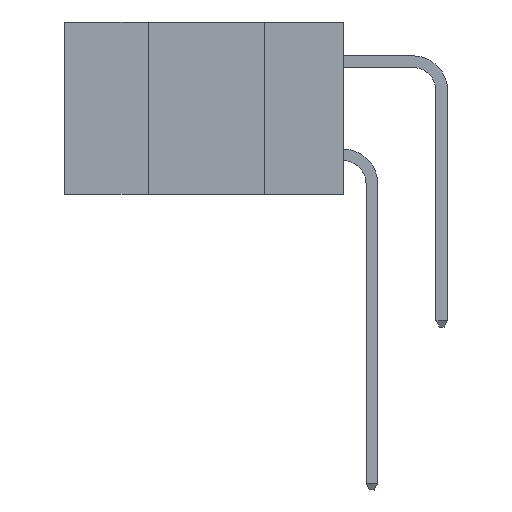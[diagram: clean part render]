
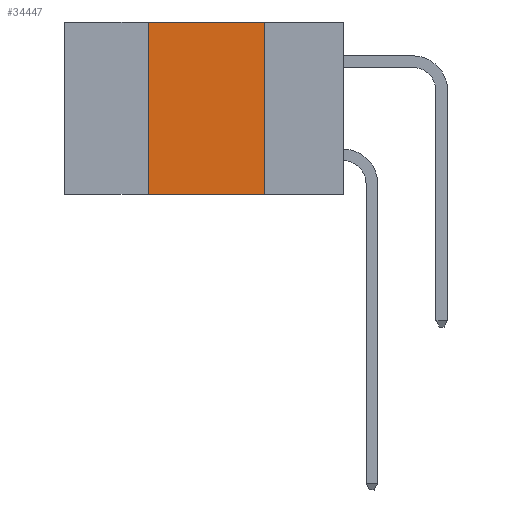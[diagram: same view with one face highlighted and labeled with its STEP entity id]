
A CAD part, left-side view. The second image highlights one B-rep face of the part: STEP entity #34447.
In plain terms, the highlighted planar face has unit normal (-1, 0, 0).
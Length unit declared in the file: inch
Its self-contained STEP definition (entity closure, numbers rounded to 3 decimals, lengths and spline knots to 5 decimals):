
#1745 = EDGE_LOOP ( 'NONE', ( #3481, #4021, #26736, #11345 ) ) ;
#1774 = VECTOR ( 'NONE', #10986, 39.37008 ) ;
#2614 = CARTESIAN_POINT ( 'NONE',  ( 0., 0.17, 0. ) ) ;
#2617 = LINE ( 'NONE', #21585, #1774 ) ;
#3481 = ORIENTED_EDGE ( 'NONE', *, *, #29545, .F. ) ;
#3507 = CARTESIAN_POINT ( 'NONE',  ( 0., 0.6, -0.37 ) ) ;
#4021 = ORIENTED_EDGE ( 'NONE', *, *, #13967, .F. ) ;
#5089 = CARTESIAN_POINT ( 'NONE',  ( 0., 0.6, 0. ) ) ;
#5831 = DIRECTION ( 'NONE',  ( 0., 0., 1. ) ) ;
#6298 = AXIS2_PLACEMENT_3D ( 'NONE', #5089, #23743, #7770 ) ;
#7740 = VECTOR ( 'NONE', #5831, 39.37008 ) ;
#7770 = DIRECTION ( 'NONE',  ( 0., 0., -1. ) ) ;
#8889 = DIRECTION ( 'NONE',  ( 0., -1., 0. ) ) ;
#9100 = LINE ( 'NONE', #23725, #22451 ) ;
#10986 = DIRECTION ( 'NONE',  ( 0., -1., 0. ) ) ;
#11227 = FACE_OUTER_BOUND ( 'NONE', #1745, .T. ) ;
#11345 = ORIENTED_EDGE ( 'NONE', *, *, #29816, .T. ) ;
#13967 = EDGE_CURVE ( 'NONE', #16771, #19937, #2617, .T. ) ;
#15769 = PLANE ( 'NONE',  #6298 ) ;
#16771 = VERTEX_POINT ( 'NONE', #17739 ) ;
#16963 = CARTESIAN_POINT ( 'NONE',  ( 0., 0.42, -0.37 ) ) ;
#17739 = CARTESIAN_POINT ( 'NONE',  ( 0., 0.42, 0. ) ) ;
#19587 = CARTESIAN_POINT ( 'NONE',  ( 0., 0.17, -0.37 ) ) ;
#19937 = VERTEX_POINT ( 'NONE', #2614 ) ;
#21205 = LINE ( 'NONE', #3507, #34406 ) ;
#21585 = CARTESIAN_POINT ( 'NONE',  ( 0., 0.6, 0. ) ) ;
#21799 = CARTESIAN_POINT ( 'NONE',  ( 0., 0.42, 0. ) ) ;
#22451 = VECTOR ( 'NONE', #34314, 39.37008 ) ;
#23362 = VERTEX_POINT ( 'NONE', #19587 ) ;
#23725 = CARTESIAN_POINT ( 'NONE',  ( 0., 0.17, 0. ) ) ;
#23743 = DIRECTION ( 'NONE',  ( 1., 0., 0. ) ) ;
#26736 = ORIENTED_EDGE ( 'NONE', *, *, #31062, .F. ) ;
#29019 = LINE ( 'NONE', #21799, #7740 ) ;
#29545 = EDGE_CURVE ( 'NONE', #19937, #23362, #9100, .T. ) ;
#29816 = EDGE_CURVE ( 'NONE', #34092, #23362, #21205, .T. ) ;
#31062 = EDGE_CURVE ( 'NONE', #34092, #16771, #29019, .T. ) ;
#34092 = VERTEX_POINT ( 'NONE', #16963 ) ;
#34314 = DIRECTION ( 'NONE',  ( 0., 0., -1. ) ) ;
#34406 = VECTOR ( 'NONE', #8889, 39.37008 ) ;
#34447 = ADVANCED_FACE ( 'NONE', ( #11227 ), #15769, .F. ) ;
